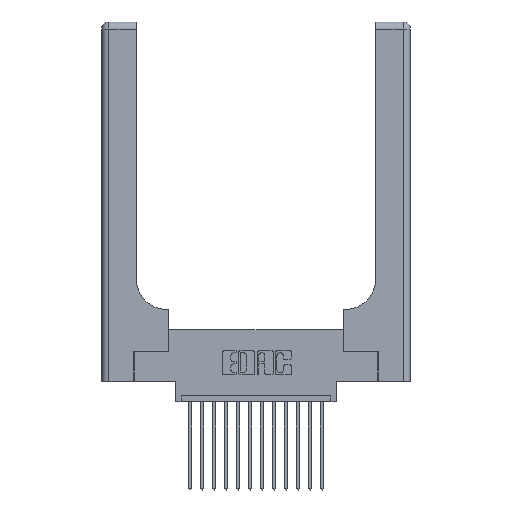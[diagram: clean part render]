
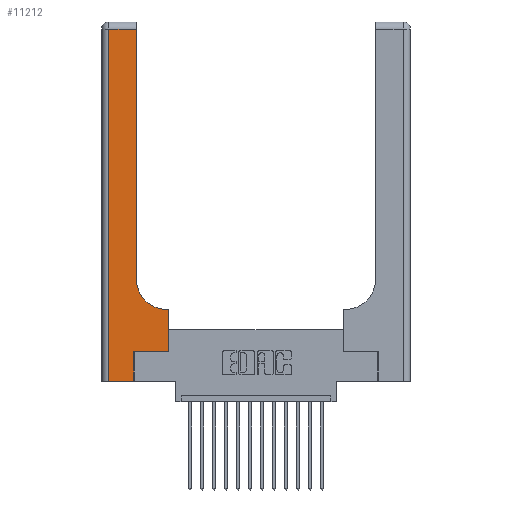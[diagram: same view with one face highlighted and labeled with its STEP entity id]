
A CAD part, top view. The second image highlights one B-rep face of the part: STEP entity #11212.
In plain terms, the highlighted planar face has unit normal (0, 0, 1).
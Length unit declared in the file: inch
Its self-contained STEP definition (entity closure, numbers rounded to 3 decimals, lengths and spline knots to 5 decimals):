
#52 = DIRECTION ( 'NONE',  ( 1., 0., 0. ) ) ;
#131 = EDGE_CURVE ( 'NONE', #6541, #229, #5037, .T. ) ;
#229 = VERTEX_POINT ( 'NONE', #2081 ) ;
#843 = LINE ( 'NONE', #13723, #4655 ) ;
#1013 = EDGE_CURVE ( 'NONE', #10669, #8213, #13048, .T. ) ;
#1732 = EDGE_LOOP ( 'NONE', ( #6227, #12266, #18398, #13913, #11758, #15157, #12730, #8211, #5308 ) ) ;
#1816 = CARTESIAN_POINT ( 'NONE',  ( 0., 2.94, 0.37 ) ) ;
#2081 = CARTESIAN_POINT ( 'NONE',  ( 0.269, 0.25, 0.37 ) ) ;
#2193 = CARTESIAN_POINT ( 'NONE',  ( 0.5585, 0.6, 0.37 ) ) ;
#2280 = EDGE_CURVE ( 'NONE', #10870, #10669, #2733, .T. ) ;
#2501 = CARTESIAN_POINT ( 'NONE',  ( 0.06, 0., 0.37 ) ) ;
#2733 = CIRCLE ( 'NONE', #11188, 0.25 ) ;
#2818 = CARTESIAN_POINT ( 'NONE',  ( 0.269, 0., 0.37 ) ) ;
#2910 = DIRECTION ( 'NONE',  ( 0., 1., 0. ) ) ;
#3110 = CARTESIAN_POINT ( 'NONE',  ( 0.2915, 0.6, 0.37 ) ) ;
#3444 = PLANE ( 'NONE',  #7409 ) ;
#4045 = EDGE_CURVE ( 'NONE', #11810, #10870, #14462, .T. ) ;
#4257 = CARTESIAN_POINT ( 'NONE',  ( 0.2915, 2.94, 0.37 ) ) ;
#4655 = VECTOR ( 'NONE', #18003, 39.37008 ) ;
#4882 = LINE ( 'NONE', #13715, #9143 ) ;
#4912 = VECTOR ( 'NONE', #17244, 39.37008 ) ;
#4949 = DIRECTION ( 'NONE',  ( -1., 0., 0. ) ) ;
#5037 = LINE ( 'NONE', #2818, #13709 ) ;
#5308 = ORIENTED_EDGE ( 'NONE', *, *, #2280, .T. ) ;
#5326 = VERTEX_POINT ( 'NONE', #15779 ) ;
#5533 = VECTOR ( 'NONE', #2910, 39.37008 ) ;
#6227 = ORIENTED_EDGE ( 'NONE', *, *, #1013, .T. ) ;
#6541 = VERTEX_POINT ( 'NONE', #12633 ) ;
#7076 = LINE ( 'NONE', #17330, #14886 ) ;
#7409 = AXIS2_PLACEMENT_3D ( 'NONE', #7794, #10518, #4949 ) ;
#7561 = CARTESIAN_POINT ( 'NONE',  ( 0.2915, 3., 0.37 ) ) ;
#7775 = VERTEX_POINT ( 'NONE', #11401 ) ;
#7794 = CARTESIAN_POINT ( 'NONE',  ( 0., 3., 0.37 ) ) ;
#8211 = ORIENTED_EDGE ( 'NONE', *, *, #4045, .T. ) ;
#8213 = VERTEX_POINT ( 'NONE', #4257 ) ;
#8814 = DIRECTION ( 'NONE',  ( 0., -1., 0. ) ) ;
#9143 = VECTOR ( 'NONE', #52, 39.37008 ) ;
#9317 = EDGE_CURVE ( 'NONE', #229, #7775, #4882, .T. ) ;
#9941 = EDGE_CURVE ( 'NONE', #7775, #11810, #17096, .T. ) ;
#10518 = DIRECTION ( 'NONE',  ( 0., 0., -1. ) ) ;
#10669 = VERTEX_POINT ( 'NONE', #13263 ) ;
#10847 = CARTESIAN_POINT ( 'NONE',  ( 0.5415, 0.85, 0.37 ) ) ;
#10870 = VERTEX_POINT ( 'NONE', #11145 ) ;
#11003 = DIRECTION ( 'NONE',  ( 0., 1., 0. ) ) ;
#11145 = CARTESIAN_POINT ( 'NONE',  ( 0.5415, 0.6, 0.37 ) ) ;
#11188 = AXIS2_PLACEMENT_3D ( 'NONE', #10847, #13698, #12462 ) ;
#11212 = ADVANCED_FACE ( 'NONE', ( #11389 ), #3444, .F. ) ;
#11389 = FACE_OUTER_BOUND ( 'NONE', #1732, .T. ) ;
#11401 = CARTESIAN_POINT ( 'NONE',  ( 0.5585, 0.25, 0.37 ) ) ;
#11553 = LINE ( 'NONE', #1816, #12008 ) ;
#11758 = ORIENTED_EDGE ( 'NONE', *, *, #131, .T. ) ;
#11810 = VERTEX_POINT ( 'NONE', #2193 ) ;
#12008 = VECTOR ( 'NONE', #14674, 39.37008 ) ;
#12266 = ORIENTED_EDGE ( 'NONE', *, *, #17398, .T. ) ;
#12462 = DIRECTION ( 'NONE',  ( 1., 0., 0. ) ) ;
#12633 = CARTESIAN_POINT ( 'NONE',  ( 0.269, 0., 0.37 ) ) ;
#12730 = ORIENTED_EDGE ( 'NONE', *, *, #9941, .T. ) ;
#13048 = LINE ( 'NONE', #7561, #17703 ) ;
#13263 = CARTESIAN_POINT ( 'NONE',  ( 0.2915, 0.85, 0.37 ) ) ;
#13698 = DIRECTION ( 'NONE',  ( 0., 0., -1. ) ) ;
#13709 = VECTOR ( 'NONE', #11003, 39.37008 ) ;
#13715 = CARTESIAN_POINT ( 'NONE',  ( 0.269, 0.25, 0.37 ) ) ;
#13723 = CARTESIAN_POINT ( 'NONE',  ( 0., 0., 0.37 ) ) ;
#13913 = ORIENTED_EDGE ( 'NONE', *, *, #17083, .T. ) ;
#14462 = LINE ( 'NONE', #3110, #4912 ) ;
#14674 = DIRECTION ( 'NONE',  ( -1., 0., 0. ) ) ;
#14886 = VECTOR ( 'NONE', #8814, 39.37008 ) ;
#15157 = ORIENTED_EDGE ( 'NONE', *, *, #9317, .T. ) ;
#15485 = CARTESIAN_POINT ( 'NONE',  ( 0.5585, 0.25, 0.37 ) ) ;
#15779 = CARTESIAN_POINT ( 'NONE',  ( 0.06, 2.94, 0.37 ) ) ;
#16098 = VERTEX_POINT ( 'NONE', #2501 ) ;
#17083 = EDGE_CURVE ( 'NONE', #16098, #6541, #843, .T. ) ;
#17096 = LINE ( 'NONE', #15485, #5533 ) ;
#17244 = DIRECTION ( 'NONE',  ( -1., 0., 0. ) ) ;
#17304 = EDGE_CURVE ( 'NONE', #5326, #16098, #7076, .T. ) ;
#17330 = CARTESIAN_POINT ( 'NONE',  ( 0.06, 3., 0.37 ) ) ;
#17398 = EDGE_CURVE ( 'NONE', #8213, #5326, #11553, .T. ) ;
#17481 = DIRECTION ( 'NONE',  ( 0., 1., 0. ) ) ;
#17703 = VECTOR ( 'NONE', #17481, 39.37008 ) ;
#18003 = DIRECTION ( 'NONE',  ( 1., 0., 0. ) ) ;
#18398 = ORIENTED_EDGE ( 'NONE', *, *, #17304, .T. ) ;
